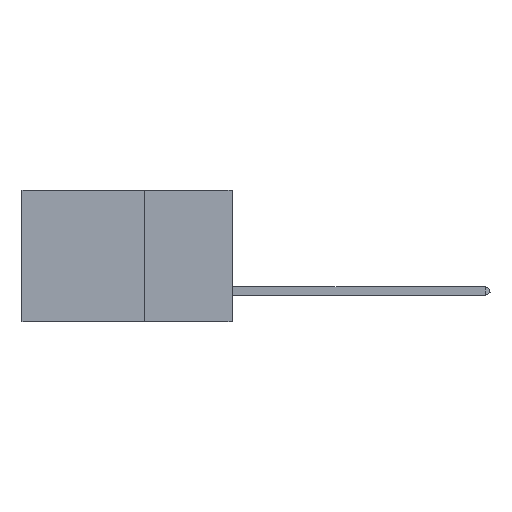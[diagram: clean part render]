
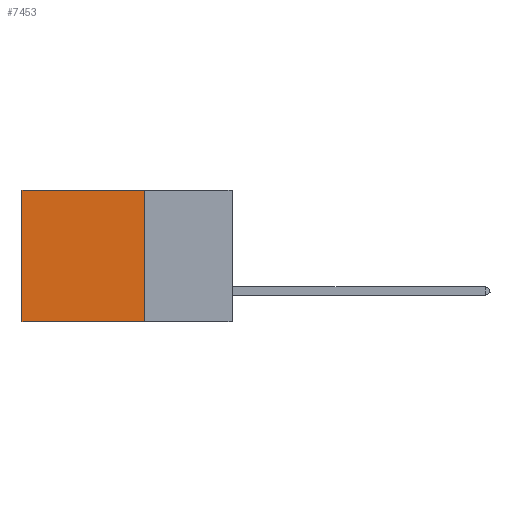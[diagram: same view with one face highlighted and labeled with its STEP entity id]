
A CAD part, left-side view. The second image highlights one B-rep face of the part: STEP entity #7453.
In plain terms, the highlighted planar face has unit normal (-1, 0, 0).
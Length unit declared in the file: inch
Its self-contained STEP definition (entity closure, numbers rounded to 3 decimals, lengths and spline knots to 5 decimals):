
#110 = EDGE_CURVE ( 'NONE', #14609, #11669, #5557, .T. ) ;
#360 = CARTESIAN_POINT ( 'NONE',  ( 0.2875, 0.6, -0.375 ) ) ;
#410 = PLANE ( 'NONE',  #10858 ) ;
#914 = ORIENTED_EDGE ( 'NONE', *, *, #12789, .T. ) ;
#1651 = VERTEX_POINT ( 'NONE', #10428 ) ;
#2435 = EDGE_CURVE ( 'NONE', #14609, #1651, #14843, .T. ) ;
#2821 = ORIENTED_EDGE ( 'NONE', *, *, #6924, .F. ) ;
#2977 = CARTESIAN_POINT ( 'NONE',  ( 0.2875, 0.25, -0.375 ) ) ;
#3786 = DIRECTION ( 'NONE',  ( 0., 1., 0. ) ) ;
#4017 = CARTESIAN_POINT ( 'NONE',  ( 0.2875, 0.6, 0. ) ) ;
#4102 = CARTESIAN_POINT ( 'NONE',  ( 0.2875, 0.25, -0.375 ) ) ;
#4221 = ORIENTED_EDGE ( 'NONE', *, *, #110, .T. ) ;
#4242 = ORIENTED_EDGE ( 'NONE', *, *, #2435, .F. ) ;
#4936 = DIRECTION ( 'NONE',  ( 0., 0., -1. ) ) ;
#5139 = DIRECTION ( 'NONE',  ( 1., 0., 0. ) ) ;
#5557 = LINE ( 'NONE', #7436, #7538 ) ;
#6101 = LINE ( 'NONE', #360, #8284 ) ;
#6820 = EDGE_LOOP ( 'NONE', ( #914, #2821, #4242, #4221 ) ) ;
#6924 = EDGE_CURVE ( 'NONE', #1651, #14084, #12421, .T. ) ;
#7436 = CARTESIAN_POINT ( 'NONE',  ( 0.2875, 0.25, 0. ) ) ;
#7453 = ADVANCED_FACE ( 'NONE', ( #10612 ), #410, .F. ) ;
#7538 = VECTOR ( 'NONE', #3786, 39.37008 ) ;
#7732 = DIRECTION ( 'NONE',  ( 0., 1., 0. ) ) ;
#8284 = VECTOR ( 'NONE', #4936, 39.37008 ) ;
#8493 = CARTESIAN_POINT ( 'NONE',  ( 0.2875, 0.25, -0.375 ) ) ;
#8628 = DIRECTION ( 'NONE',  ( 0., 0., -1. ) ) ;
#10428 = CARTESIAN_POINT ( 'NONE',  ( 0.2875, 0.25, -0.375 ) ) ;
#10522 = CARTESIAN_POINT ( 'NONE',  ( 0.2875, 0.25, 0. ) ) ;
#10544 = CARTESIAN_POINT ( 'NONE',  ( 0.2875, 0.6, -0.375 ) ) ;
#10612 = FACE_OUTER_BOUND ( 'NONE', #6820, .T. ) ;
#10858 = AXIS2_PLACEMENT_3D ( 'NONE', #8493, #5139, #14389 ) ;
#11669 = VERTEX_POINT ( 'NONE', #4017 ) ;
#12060 = VECTOR ( 'NONE', #7732, 39.37008 ) ;
#12421 = LINE ( 'NONE', #2977, #12060 ) ;
#12789 = EDGE_CURVE ( 'NONE', #11669, #14084, #6101, .T. ) ;
#13967 = VECTOR ( 'NONE', #8628, 39.37008 ) ;
#14084 = VERTEX_POINT ( 'NONE', #10544 ) ;
#14389 = DIRECTION ( 'NONE',  ( 0., 0., -1. ) ) ;
#14609 = VERTEX_POINT ( 'NONE', #10522 ) ;
#14843 = LINE ( 'NONE', #4102, #13967 ) ;
